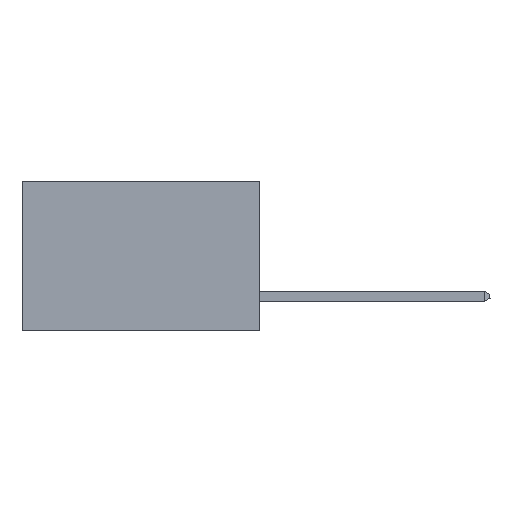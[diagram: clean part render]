
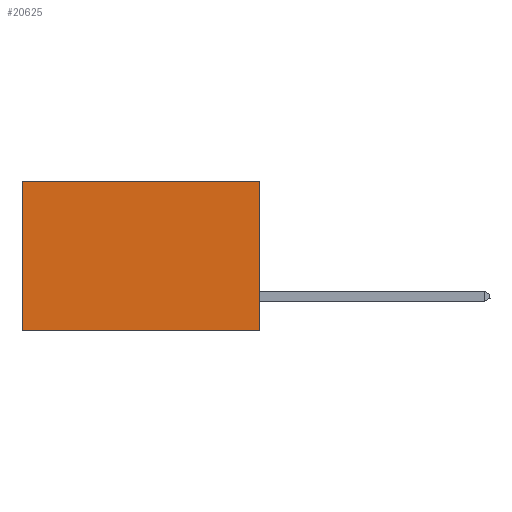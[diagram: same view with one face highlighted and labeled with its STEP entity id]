
A CAD part, left-side view. The second image highlights one B-rep face of the part: STEP entity #20625.
In plain terms, the highlighted planar face has unit normal (-1, 0, 0).
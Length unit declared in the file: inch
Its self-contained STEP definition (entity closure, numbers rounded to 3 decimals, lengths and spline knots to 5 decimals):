
#97 = DIRECTION ( 'NONE',  ( 1., 0., 0. ) ) ;
#1002 = CARTESIAN_POINT ( 'NONE',  ( 0.277, 0.59, 0. ) ) ;
#1856 = DIRECTION ( 'NONE',  ( 0., 1., 0. ) ) ;
#2754 = EDGE_LOOP ( 'NONE', ( #25292, #11981, #3050, #25962 ) ) ;
#3050 = ORIENTED_EDGE ( 'NONE', *, *, #10401, .F. ) ;
#3449 = AXIS2_PLACEMENT_3D ( 'NONE', #24359, #97, #14235 ) ;
#5204 = VERTEX_POINT ( 'NONE', #1002 ) ;
#7299 = CARTESIAN_POINT ( 'NONE',  ( 0.277, 0.59, -0.37 ) ) ;
#9644 = VECTOR ( 'NONE', #17100, 39.37008 ) ;
#10117 = VERTEX_POINT ( 'NONE', #22339 ) ;
#10162 = PLANE ( 'NONE',  #3449 ) ;
#10189 = FACE_OUTER_BOUND ( 'NONE', #2754, .T. ) ;
#10401 = EDGE_CURVE ( 'NONE', #10117, #21475, #15038, .T. ) ;
#11057 = CARTESIAN_POINT ( 'NONE',  ( 0.277, 0., -0.37 ) ) ;
#11662 = LINE ( 'NONE', #23951, #21857 ) ;
#11981 = ORIENTED_EDGE ( 'NONE', *, *, #15085, .F. ) ;
#12904 = LINE ( 'NONE', #18042, #22460 ) ;
#13385 = VECTOR ( 'NONE', #17388, 39.37008 ) ;
#14023 = LINE ( 'NONE', #7299, #13385 ) ;
#14111 = CARTESIAN_POINT ( 'NONE',  ( 0.277, 0.59, -0.37 ) ) ;
#14235 = DIRECTION ( 'NONE',  ( 0., 0., -1. ) ) ;
#15038 = LINE ( 'NONE', #11057, #9644 ) ;
#15085 = EDGE_CURVE ( 'NONE', #21475, #19214, #11662, .T. ) ;
#17100 = DIRECTION ( 'NONE',  ( 0., 0., -1. ) ) ;
#17388 = DIRECTION ( 'NONE',  ( 0., 0., -1. ) ) ;
#17923 = CARTESIAN_POINT ( 'NONE',  ( 0.277, 0., -0.37 ) ) ;
#18042 = CARTESIAN_POINT ( 'NONE',  ( 0.277, 0., 0. ) ) ;
#19214 = VERTEX_POINT ( 'NONE', #14111 ) ;
#20625 = ADVANCED_FACE ( 'NONE', ( #10189 ), #10162, .F. ) ;
#21475 = VERTEX_POINT ( 'NONE', #17923 ) ;
#21857 = VECTOR ( 'NONE', #25916, 39.37008 ) ;
#22339 = CARTESIAN_POINT ( 'NONE',  ( 0.277, 0., 0. ) ) ;
#22460 = VECTOR ( 'NONE', #1856, 39.37008 ) ;
#22845 = EDGE_CURVE ( 'NONE', #10117, #5204, #12904, .T. ) ;
#23951 = CARTESIAN_POINT ( 'NONE',  ( 0.277, 0., -0.37 ) ) ;
#24359 = CARTESIAN_POINT ( 'NONE',  ( 0.277, 0., -0.37 ) ) ;
#25292 = ORIENTED_EDGE ( 'NONE', *, *, #25749, .T. ) ;
#25749 = EDGE_CURVE ( 'NONE', #5204, #19214, #14023, .T. ) ;
#25916 = DIRECTION ( 'NONE',  ( 0., 1., 0. ) ) ;
#25962 = ORIENTED_EDGE ( 'NONE', *, *, #22845, .T. ) ;
